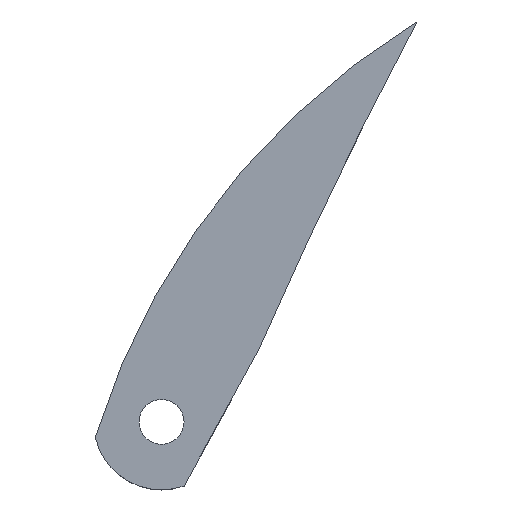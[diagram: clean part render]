
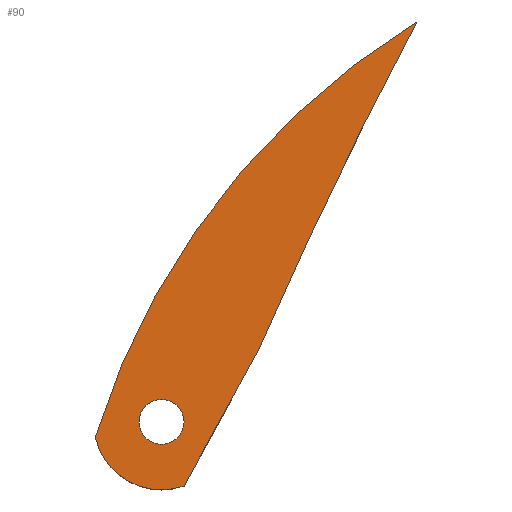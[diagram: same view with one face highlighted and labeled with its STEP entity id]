
A CAD part, top view. The second image highlights one B-rep face of the part: STEP entity #90.
In plain terms, the highlighted planar face has unit normal (0, 0, 1).
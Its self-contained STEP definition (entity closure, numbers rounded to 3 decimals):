
#1 = EDGE_CURVE ( 'NONE', #5, #252, #193, .T. ) ;
#2 = DIRECTION ( 'NONE',  ( 0., 0., 1. ) ) ;
#3 = CIRCLE ( 'NONE', #13, 6.051 ) ;
#5 = VERTEX_POINT ( 'NONE', #154 ) ;
#13 = AXIS2_PLACEMENT_3D ( 'NONE', #26, #2, #187 ) ;
#16 = CARTESIAN_POINT ( 'NONE',  ( 0., 0., 6. ) ) ;
#22 = ORIENTED_EDGE ( 'NONE', *, *, #204, .F. ) ;
#26 = CARTESIAN_POINT ( 'NONE',  ( 0., 0., 6. ) ) ;
#27 = ORIENTED_EDGE ( 'NONE', *, *, #1, .T. ) ;
#28 = VERTEX_POINT ( 'NONE', #47 ) ;
#31 = EDGE_CURVE ( 'NONE', #252, #246, #3, .T. ) ;
#33 = CARTESIAN_POINT ( 'NONE',  ( 57.298, -20.763, 6. ) ) ;
#36 = CARTESIAN_POINT ( 'NONE',  ( 8.646, 6.405, 6. ) ) ;
#37 = DIRECTION ( 'NONE',  ( -1., 0., 0. ) ) ;
#41 = ORIENTED_EDGE ( 'NONE', *, *, #158, .T. ) ;
#42 = DIRECTION ( 'NONE',  ( 0., 0., -1. ) ) ;
#47 = CARTESIAN_POINT ( 'NONE',  ( 8.646, 6.405, 6. ) ) ;
#49 = AXIS2_PLACEMENT_3D ( 'NONE', #112, #68, #150 ) ;
#57 = DIRECTION ( 'NONE',  ( 1., 0., 0. ) ) ;
#66 = EDGE_LOOP ( 'NONE', ( #27, #243, #256, #41 ) ) ;
#68 = DIRECTION ( 'NONE',  ( 0., 0., 1. ) ) ;
#77 = DIRECTION ( 'NONE',  ( 0.481, 0.877, 0. ) ) ;
#79 = EDGE_LOOP ( 'NONE', ( #212, #22 ) ) ;
#90 = ADVANCED_FACE ( 'NONE', ( #92, #140 ), #261, .F. ) ;
#92 = FACE_OUTER_BOUND ( 'NONE', #66, .T. ) ;
#98 = EDGE_CURVE ( 'NONE', #236, #165, #239, .T. ) ;
#107 = AXIS2_PLACEMENT_3D ( 'NONE', #33, #219, #157 ) ;
#112 = CARTESIAN_POINT ( 'NONE',  ( 57.298, -20.763, 6. ) ) ;
#118 = CIRCLE ( 'NONE', #221, 2. ) ;
#124 = CARTESIAN_POINT ( 'NONE',  ( 2., -5.711, 6. ) ) ;
#125 = CIRCLE ( 'NONE', #160, 425.046 ) ;
#140 = FACE_BOUND ( 'NONE', #79, .T. ) ;
#142 = CARTESIAN_POINT ( 'NONE',  ( -2., 0., 6. ) ) ;
#150 = DIRECTION ( 'NONE',  ( -1., 0., 0. ) ) ;
#154 = CARTESIAN_POINT ( 'NONE',  ( 22.692, 35.547, 6. ) ) ;
#157 = DIRECTION ( 'NONE',  ( -1., 0., 0. ) ) ;
#158 = EDGE_CURVE ( 'NONE', #28, #5, #125, .T. ) ;
#160 = AXIS2_PLACEMENT_3D ( 'NONE', #227, #42, #37 ) ;
#162 = CARTESIAN_POINT ( 'NONE',  ( -5.891, -1.383, 6. ) ) ;
#165 = VERTEX_POINT ( 'NONE', #180 ) ;
#180 = CARTESIAN_POINT ( 'NONE',  ( 2., 0., 6. ) ) ;
#183 = DIRECTION ( 'NONE',  ( 1., 0., 0. ) ) ;
#187 = DIRECTION ( 'NONE',  ( -1., 0., 0. ) ) ;
#193 = CIRCLE ( 'NONE', #49, 66.094 ) ;
#204 = EDGE_CURVE ( 'NONE', #165, #236, #118, .T. ) ;
#212 = ORIENTED_EDGE ( 'NONE', *, *, #98, .F. ) ;
#213 = VECTOR ( 'NONE', #77, 1000. ) ;
#219 = DIRECTION ( 'NONE',  ( 0., 0., -1. ) ) ;
#221 = AXIS2_PLACEMENT_3D ( 'NONE', #265, #247, #183 ) ;
#227 = CARTESIAN_POINT ( 'NONE',  ( 398.281, -163.442, 6. ) ) ;
#236 = VERTEX_POINT ( 'NONE', #142 ) ;
#239 = CIRCLE ( 'NONE', #267, 2. ) ;
#240 = DIRECTION ( 'NONE',  ( 0., 0., 1. ) ) ;
#243 = ORIENTED_EDGE ( 'NONE', *, *, #31, .T. ) ;
#246 = VERTEX_POINT ( 'NONE', #124 ) ;
#247 = DIRECTION ( 'NONE',  ( 0., 0., 1. ) ) ;
#252 = VERTEX_POINT ( 'NONE', #162 ) ;
#253 = EDGE_CURVE ( 'NONE', #246, #28, #263, .T. ) ;
#256 = ORIENTED_EDGE ( 'NONE', *, *, #253, .T. ) ;
#261 = PLANE ( 'NONE',  #107 ) ;
#263 = LINE ( 'NONE', #36, #213 ) ;
#265 = CARTESIAN_POINT ( 'NONE',  ( 0., 0., 6. ) ) ;
#267 = AXIS2_PLACEMENT_3D ( 'NONE', #16, #240, #57 ) ;
